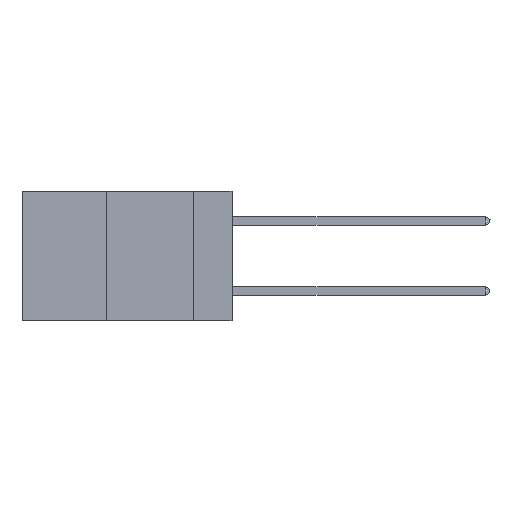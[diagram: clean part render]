
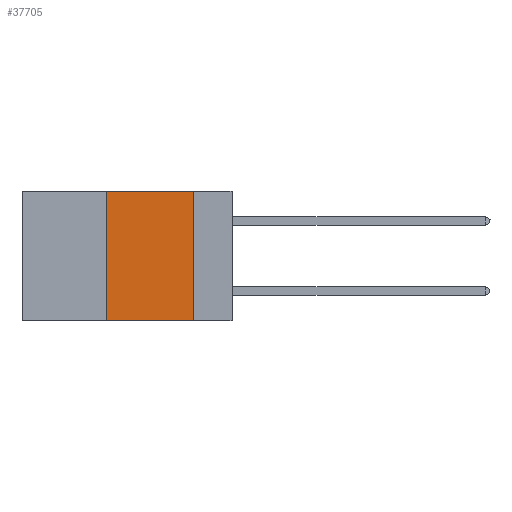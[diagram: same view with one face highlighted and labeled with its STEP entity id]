
A CAD part, left-side view. The second image highlights one B-rep face of the part: STEP entity #37705.
In plain terms, the highlighted planar face has unit normal (-1, 0, 0).
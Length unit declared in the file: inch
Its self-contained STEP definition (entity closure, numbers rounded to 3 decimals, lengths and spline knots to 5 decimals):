
#2702 = CARTESIAN_POINT ( 'NONE',  ( 0., 0.36, 0. ) ) ;
#3804 = DIRECTION ( 'NONE',  ( 0., 0., -1. ) ) ;
#4333 = ORIENTED_EDGE ( 'NONE', *, *, #26202, .F. ) ;
#4612 = PLANE ( 'NONE',  #24479 ) ;
#5907 = LINE ( 'NONE', #10337, #30523 ) ;
#7870 = DIRECTION ( 'NONE',  ( 1., 0., 0. ) ) ;
#9205 = LINE ( 'NONE', #2702, #33706 ) ;
#10337 = CARTESIAN_POINT ( 'NONE',  ( 0., 0.11, 0. ) ) ;
#10389 = CARTESIAN_POINT ( 'NONE',  ( 0., 0.6, 0. ) ) ;
#11490 = CARTESIAN_POINT ( 'NONE',  ( 0., 0.36, 0. ) ) ;
#13041 = ORIENTED_EDGE ( 'NONE', *, *, #26986, .T. ) ;
#13226 = CARTESIAN_POINT ( 'NONE',  ( 0., 0.36, -0.37 ) ) ;
#15745 = CARTESIAN_POINT ( 'NONE',  ( 0., 0.6, -0.37 ) ) ;
#17340 = EDGE_LOOP ( 'NONE', ( #20476, #36831, #4333, #13041 ) ) ;
#19485 = FACE_OUTER_BOUND ( 'NONE', #17340, .T. ) ;
#19630 = VERTEX_POINT ( 'NONE', #11490 ) ;
#20476 = ORIENTED_EDGE ( 'NONE', *, *, #38875, .F. ) ;
#21301 = VECTOR ( 'NONE', #25363, 39.37008 ) ;
#22060 = VERTEX_POINT ( 'NONE', #30460 ) ;
#23592 = VECTOR ( 'NONE', #38920, 39.37008 ) ;
#24479 = AXIS2_PLACEMENT_3D ( 'NONE', #27111, #7870, #30326 ) ;
#24493 = VERTEX_POINT ( 'NONE', #36179 ) ;
#25363 = DIRECTION ( 'NONE',  ( 0., -1., 0. ) ) ;
#26202 = EDGE_CURVE ( 'NONE', #28558, #19630, #9205, .T. ) ;
#26986 = EDGE_CURVE ( 'NONE', #28558, #24493, #29786, .T. ) ;
#27111 = CARTESIAN_POINT ( 'NONE',  ( 0., 0.6, 0. ) ) ;
#28343 = DIRECTION ( 'NONE',  ( 0., 0., 1. ) ) ;
#28558 = VERTEX_POINT ( 'NONE', #13226 ) ;
#29786 = LINE ( 'NONE', #15745, #21301 ) ;
#30326 = DIRECTION ( 'NONE',  ( 0., 0., -1. ) ) ;
#30460 = CARTESIAN_POINT ( 'NONE',  ( 0., 0.11, 0. ) ) ;
#30523 = VECTOR ( 'NONE', #3804, 39.37008 ) ;
#33706 = VECTOR ( 'NONE', #28343, 39.37008 ) ;
#36179 = CARTESIAN_POINT ( 'NONE',  ( 0., 0.11, -0.37 ) ) ;
#36831 = ORIENTED_EDGE ( 'NONE', *, *, #38239, .F. ) ;
#37705 = ADVANCED_FACE ( 'NONE', ( #19485 ), #4612, .F. ) ;
#38239 = EDGE_CURVE ( 'NONE', #19630, #22060, #38426, .T. ) ;
#38426 = LINE ( 'NONE', #10389, #23592 ) ;
#38875 = EDGE_CURVE ( 'NONE', #22060, #24493, #5907, .T. ) ;
#38920 = DIRECTION ( 'NONE',  ( 0., -1., 0. ) ) ;
